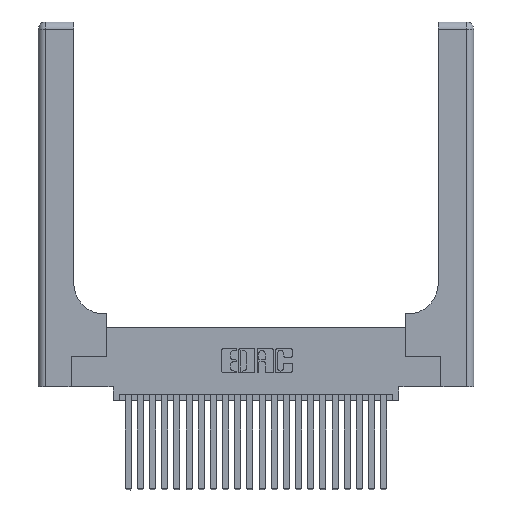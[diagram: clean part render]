
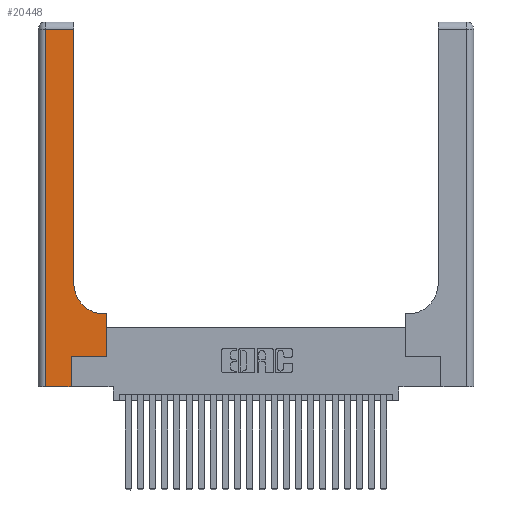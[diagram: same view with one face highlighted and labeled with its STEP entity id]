
A CAD part, top view. The second image highlights one B-rep face of the part: STEP entity #20448.
In plain terms, the highlighted planar face has unit normal (0, 0, 1).
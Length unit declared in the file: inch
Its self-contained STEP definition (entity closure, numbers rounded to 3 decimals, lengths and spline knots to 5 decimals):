
#584 = DIRECTION ( 'NONE',  ( 0., 1., 0. ) ) ;
#754 = CARTESIAN_POINT ( 'NONE',  ( 0.5585, 0.25, 0.37 ) ) ;
#930 = ORIENTED_EDGE ( 'NONE', *, *, #18045, .T. ) ;
#1105 = VERTEX_POINT ( 'NONE', #20138 ) ;
#1812 = CARTESIAN_POINT ( 'NONE',  ( 0.2915, 0.85, 0.37 ) ) ;
#1814 = VECTOR ( 'NONE', #11541, 39.37008 ) ;
#1973 = CARTESIAN_POINT ( 'NONE',  ( 0.269, 0., 0.37 ) ) ;
#2172 = EDGE_CURVE ( 'NONE', #14791, #19368, #23081, .T. ) ;
#2400 = EDGE_CURVE ( 'NONE', #12659, #7456, #22755, .T. ) ;
#2871 = ORIENTED_EDGE ( 'NONE', *, *, #17782, .T. ) ;
#3922 = ORIENTED_EDGE ( 'NONE', *, *, #15196, .T. ) ;
#4117 = CARTESIAN_POINT ( 'NONE',  ( 0., 2.94, 0.37 ) ) ;
#4251 = ORIENTED_EDGE ( 'NONE', *, *, #22691, .T. ) ;
#5183 = VECTOR ( 'NONE', #14625, 39.37008 ) ;
#5923 = CARTESIAN_POINT ( 'NONE',  ( 0.269, 0., 0.37 ) ) ;
#6228 = DIRECTION ( 'NONE',  ( 1., 0., 0. ) ) ;
#7136 = VERTEX_POINT ( 'NONE', #1812 ) ;
#7456 = VERTEX_POINT ( 'NONE', #22487 ) ;
#7733 = EDGE_LOOP ( 'NONE', ( #2871, #3922, #12748, #14670, #18499, #13523, #18206, #4251, #930 ) ) ;
#9322 = VECTOR ( 'NONE', #24949, 39.37008 ) ;
#9469 = DIRECTION ( 'NONE',  ( 0., 0., -1. ) ) ;
#9900 = EDGE_CURVE ( 'NONE', #7456, #22179, #11700, .T. ) ;
#9949 = CARTESIAN_POINT ( 'NONE',  ( 0.06, 2.94, 0.37 ) ) ;
#10079 = DIRECTION ( 'NONE',  ( 1., 0., 0. ) ) ;
#10288 = LINE ( 'NONE', #21225, #9322 ) ;
#11541 = DIRECTION ( 'NONE',  ( 0., 1., 0. ) ) ;
#11700 = LINE ( 'NONE', #15329, #11985 ) ;
#11751 = DIRECTION ( 'NONE',  ( 0., 0., -1. ) ) ;
#11876 = VECTOR ( 'NONE', #10079, 39.37008 ) ;
#11953 = CARTESIAN_POINT ( 'NONE',  ( 0.269, 0.25, 0.37 ) ) ;
#11985 = VECTOR ( 'NONE', #6228, 39.37008 ) ;
#12610 = VERTEX_POINT ( 'NONE', #17479 ) ;
#12659 = VERTEX_POINT ( 'NONE', #9949 ) ;
#12748 = ORIENTED_EDGE ( 'NONE', *, *, #2400, .T. ) ;
#13523 = ORIENTED_EDGE ( 'NONE', *, *, #2172, .T. ) ;
#14003 = LINE ( 'NONE', #5923, #1814 ) ;
#14625 = DIRECTION ( 'NONE',  ( 0., -1., 0. ) ) ;
#14670 = ORIENTED_EDGE ( 'NONE', *, *, #9900, .T. ) ;
#14761 = LINE ( 'NONE', #754, #18997 ) ;
#14791 = VERTEX_POINT ( 'NONE', #23821 ) ;
#14845 = AXIS2_PLACEMENT_3D ( 'NONE', #17423, #9469, #19051 ) ;
#15196 = EDGE_CURVE ( 'NONE', #24268, #12659, #16632, .T. ) ;
#15329 = CARTESIAN_POINT ( 'NONE',  ( 0., 0., 0.37 ) ) ;
#15816 = CARTESIAN_POINT ( 'NONE',  ( 0., 3., 0.37 ) ) ;
#16028 = CARTESIAN_POINT ( 'NONE',  ( 0.2915, 3., 0.37 ) ) ;
#16632 = LINE ( 'NONE', #4117, #24208 ) ;
#16773 = LINE ( 'NONE', #16028, #20398 ) ;
#16908 = CARTESIAN_POINT ( 'NONE',  ( 0.2915, 2.94, 0.37 ) ) ;
#17412 = EDGE_CURVE ( 'NONE', #19368, #12610, #14761, .T. ) ;
#17423 = CARTESIAN_POINT ( 'NONE',  ( 0.5415, 0.85, 0.37 ) ) ;
#17479 = CARTESIAN_POINT ( 'NONE',  ( 0.5585, 0.6, 0.37 ) ) ;
#17514 = DIRECTION ( 'NONE',  ( -1., 0., 0. ) ) ;
#17782 = EDGE_CURVE ( 'NONE', #7136, #24268, #16773, .T. ) ;
#18045 = EDGE_CURVE ( 'NONE', #1105, #7136, #18979, .T. ) ;
#18206 = ORIENTED_EDGE ( 'NONE', *, *, #17412, .T. ) ;
#18226 = DIRECTION ( 'NONE',  ( 0., 1., 0. ) ) ;
#18499 = ORIENTED_EDGE ( 'NONE', *, *, #21513, .T. ) ;
#18979 = CIRCLE ( 'NONE', #14845, 0.25 ) ;
#18997 = VECTOR ( 'NONE', #18226, 39.37008 ) ;
#19051 = DIRECTION ( 'NONE',  ( 1., 0., 0. ) ) ;
#19368 = VERTEX_POINT ( 'NONE', #24926 ) ;
#19534 = DIRECTION ( 'NONE',  ( -1., 0., 0. ) ) ;
#19628 = PLANE ( 'NONE',  #21359 ) ;
#20138 = CARTESIAN_POINT ( 'NONE',  ( 0.5415, 0.6, 0.37 ) ) ;
#20383 = CARTESIAN_POINT ( 'NONE',  ( 0.06, 3., 0.37 ) ) ;
#20398 = VECTOR ( 'NONE', #584, 39.37008 ) ;
#20448 = ADVANCED_FACE ( 'NONE', ( #22198 ), #19628, .F. ) ;
#21225 = CARTESIAN_POINT ( 'NONE',  ( 0.2915, 0.6, 0.37 ) ) ;
#21359 = AXIS2_PLACEMENT_3D ( 'NONE', #15816, #11751, #19534 ) ;
#21513 = EDGE_CURVE ( 'NONE', #22179, #14791, #14003, .T. ) ;
#22179 = VERTEX_POINT ( 'NONE', #1973 ) ;
#22198 = FACE_OUTER_BOUND ( 'NONE', #7733, .T. ) ;
#22487 = CARTESIAN_POINT ( 'NONE',  ( 0.06, 0., 0.37 ) ) ;
#22691 = EDGE_CURVE ( 'NONE', #12610, #1105, #10288, .T. ) ;
#22755 = LINE ( 'NONE', #20383, #5183 ) ;
#23081 = LINE ( 'NONE', #11953, #11876 ) ;
#23821 = CARTESIAN_POINT ( 'NONE',  ( 0.269, 0.25, 0.37 ) ) ;
#24208 = VECTOR ( 'NONE', #17514, 39.37008 ) ;
#24268 = VERTEX_POINT ( 'NONE', #16908 ) ;
#24926 = CARTESIAN_POINT ( 'NONE',  ( 0.5585, 0.25, 0.37 ) ) ;
#24949 = DIRECTION ( 'NONE',  ( -1., 0., 0. ) ) ;
